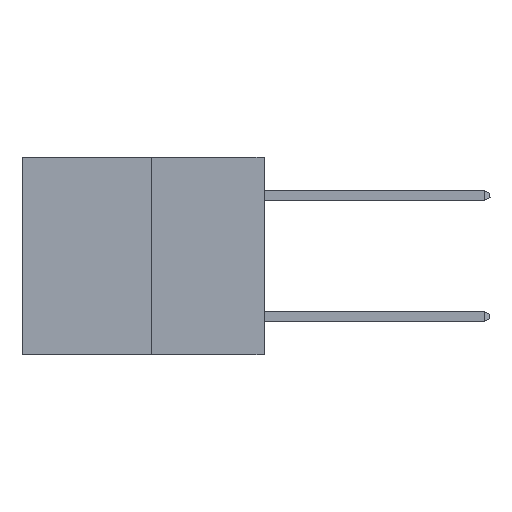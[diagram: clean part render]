
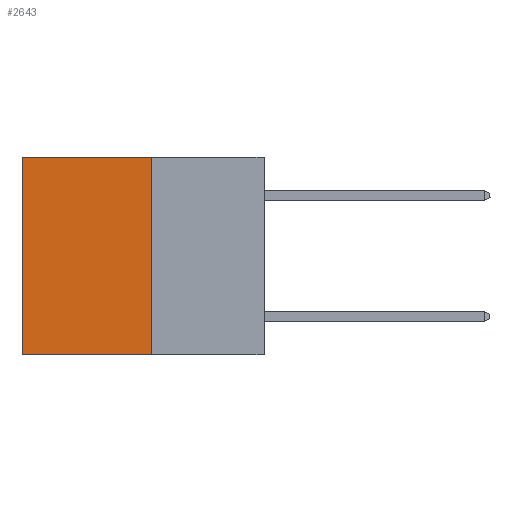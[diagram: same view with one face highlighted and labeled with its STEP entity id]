
A CAD part, left-side view. The second image highlights one B-rep face of the part: STEP entity #2643.
In plain terms, the highlighted planar face has unit normal (-1, 0, 0).
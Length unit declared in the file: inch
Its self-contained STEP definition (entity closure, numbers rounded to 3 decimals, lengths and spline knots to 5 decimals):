
#111 = DIRECTION ( 'NONE',  ( 0., 0., -1. ) ) ;
#113 = CARTESIAN_POINT ( 'NONE',  ( 0.3165, 0.28, 0. ) ) ;
#1214 = CARTESIAN_POINT ( 'NONE',  ( 0.3165, 0.28, -0.49 ) ) ;
#1969 = VERTEX_POINT ( 'NONE', #16469 ) ;
#2079 = EDGE_CURVE ( 'NONE', #1969, #2208, #14857, .T. ) ;
#2140 = ORIENTED_EDGE ( 'NONE', *, *, #13453, .F. ) ;
#2208 = VERTEX_POINT ( 'NONE', #21400 ) ;
#2600 = LINE ( 'NONE', #1214, #6099 ) ;
#2643 = ADVANCED_FACE ( 'NONE', ( #4100 ), #23139, .F. ) ;
#3178 = DIRECTION ( 'NONE',  ( 0., 0., -1. ) ) ;
#4100 = FACE_OUTER_BOUND ( 'NONE', #15784, .T. ) ;
#5131 = ORIENTED_EDGE ( 'NONE', *, *, #2079, .T. ) ;
#5585 = DIRECTION ( 'NONE',  ( 0., 1., 0. ) ) ;
#5864 = EDGE_CURVE ( 'NONE', #16604, #2208, #23966, .T. ) ;
#6099 = VECTOR ( 'NONE', #3178, 39.37008 ) ;
#7562 = CARTESIAN_POINT ( 'NONE',  ( 0.3165, 0.6, -0.49 ) ) ;
#9234 = VERTEX_POINT ( 'NONE', #14577 ) ;
#10288 = DIRECTION ( 'NONE',  ( 0., 0., -1. ) ) ;
#13082 = DIRECTION ( 'NONE',  ( 0., 1., 0. ) ) ;
#13231 = CARTESIAN_POINT ( 'NONE',  ( 0.3165, 0.28, -0.49 ) ) ;
#13453 = EDGE_CURVE ( 'NONE', #9234, #16604, #2600, .T. ) ;
#13529 = VECTOR ( 'NONE', #5585, 39.37008 ) ;
#13880 = AXIS2_PLACEMENT_3D ( 'NONE', #19503, #15599, #10288 ) ;
#14577 = CARTESIAN_POINT ( 'NONE',  ( 0.3165, 0.28, 0. ) ) ;
#14857 = LINE ( 'NONE', #7562, #21782 ) ;
#15217 = LINE ( 'NONE', #113, #22478 ) ;
#15599 = DIRECTION ( 'NONE',  ( 1., 0., 0. ) ) ;
#15784 = EDGE_LOOP ( 'NONE', ( #5131, #19301, #2140, #22268 ) ) ;
#16469 = CARTESIAN_POINT ( 'NONE',  ( 0.3165, 0.6, 0. ) ) ;
#16568 = CARTESIAN_POINT ( 'NONE',  ( 0.3165, 0.28, -0.49 ) ) ;
#16604 = VERTEX_POINT ( 'NONE', #13231 ) ;
#19301 = ORIENTED_EDGE ( 'NONE', *, *, #5864, .F. ) ;
#19503 = CARTESIAN_POINT ( 'NONE',  ( 0.3165, 0.28, -0.49 ) ) ;
#20809 = EDGE_CURVE ( 'NONE', #9234, #1969, #15217, .T. ) ;
#21400 = CARTESIAN_POINT ( 'NONE',  ( 0.3165, 0.6, -0.49 ) ) ;
#21782 = VECTOR ( 'NONE', #111, 39.37008 ) ;
#22268 = ORIENTED_EDGE ( 'NONE', *, *, #20809, .T. ) ;
#22478 = VECTOR ( 'NONE', #13082, 39.37008 ) ;
#23139 = PLANE ( 'NONE',  #13880 ) ;
#23966 = LINE ( 'NONE', #16568, #13529 ) ;
